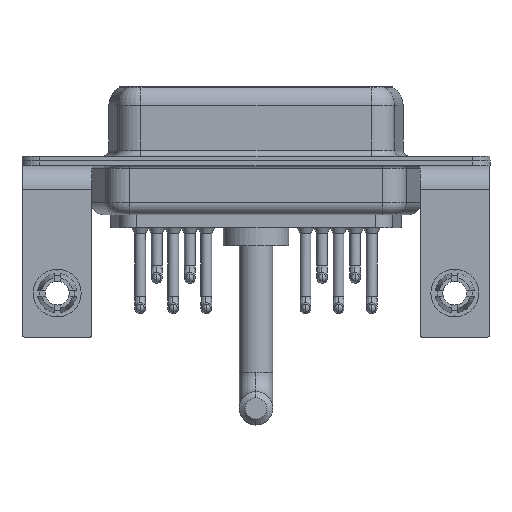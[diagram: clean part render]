
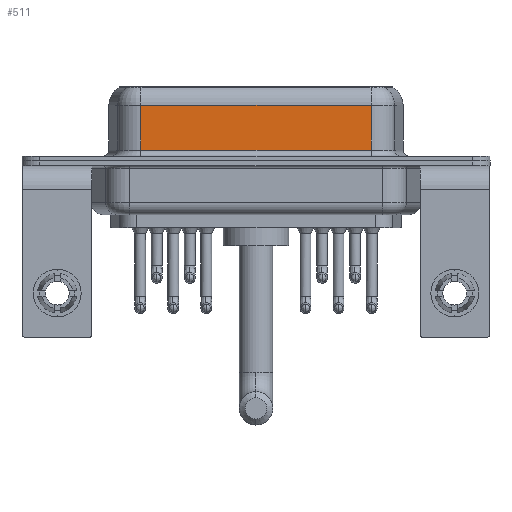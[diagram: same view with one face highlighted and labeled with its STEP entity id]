
A CAD part, front view. The second image highlights one B-rep face of the part: STEP entity #511.
In plain terms, the highlighted planar face has unit normal (0, -1, 0).
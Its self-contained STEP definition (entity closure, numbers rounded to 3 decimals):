
#489 = EDGE_CURVE ( 'NONE', #3411, #7464, #17789, .T. ) ;
#511 = ADVANCED_FACE ( 'NONE', ( #16624 ), #15010, .F. ) ;
#990 = DIRECTION ( 'NONE',  ( 0., 0., -1. ) ) ;
#3123 = CARTESIAN_POINT ( 'NONE',  ( 7.013, -3.95, 4.65 ) ) ;
#3186 = DIRECTION ( 'NONE',  ( -1., 0., 0. ) ) ;
#3411 = VERTEX_POINT ( 'NONE', #3600 ) ;
#3550 = LINE ( 'NONE', #10042, #9897 ) ;
#3600 = CARTESIAN_POINT ( 'NONE',  ( 26.287, -3.95, 4.65 ) ) ;
#4294 = CARTESIAN_POINT ( 'NONE',  ( 7.013, -3.95, 6.4 ) ) ;
#4353 = ORIENTED_EDGE ( 'NONE', *, *, #9801, .F. ) ;
#4501 = CARTESIAN_POINT ( 'NONE',  ( 26.287, -3.95, 0.9 ) ) ;
#4863 = VECTOR ( 'NONE', #18036, 1000. ) ;
#5790 = ORIENTED_EDGE ( 'NONE', *, *, #489, .T. ) ;
#6959 = CARTESIAN_POINT ( 'NONE',  ( 26.287, -3.95, 0.9 ) ) ;
#7464 = VERTEX_POINT ( 'NONE', #3123 ) ;
#9180 = VERTEX_POINT ( 'NONE', #14557 ) ;
#9801 = EDGE_CURVE ( 'NONE', #3411, #19816, #3550, .T. ) ;
#9897 = VECTOR ( 'NONE', #16562, 1000. ) ;
#9956 = VECTOR ( 'NONE', #990, 1000. ) ;
#10042 = CARTESIAN_POINT ( 'NONE',  ( 26.287, -3.95, 6.4 ) ) ;
#12236 = EDGE_LOOP ( 'NONE', ( #4353, #5790, #18954, #19613 ) ) ;
#14557 = CARTESIAN_POINT ( 'NONE',  ( 7.013, -3.95, 0.9 ) ) ;
#15010 = PLANE ( 'NONE',  #19242 ) ;
#15192 = VECTOR ( 'NONE', #3186, 1000. ) ;
#15430 = DIRECTION ( 'NONE',  ( 0., 0., 1. ) ) ;
#15496 = LINE ( 'NONE', #4294, #9956 ) ;
#16562 = DIRECTION ( 'NONE',  ( 0., 0., -1. ) ) ;
#16624 = FACE_OUTER_BOUND ( 'NONE', #12236, .T. ) ;
#16874 = LINE ( 'NONE', #6959, #4863 ) ;
#16921 = EDGE_CURVE ( 'NONE', #7464, #9180, #15496, .T. ) ;
#16940 = CARTESIAN_POINT ( 'NONE',  ( 26.287, -3.95, 6.4 ) ) ;
#17222 = EDGE_CURVE ( 'NONE', #9180, #19816, #16874, .T. ) ;
#17789 = LINE ( 'NONE', #18100, #15192 ) ;
#18036 = DIRECTION ( 'NONE',  ( 1., 0., 0. ) ) ;
#18100 = CARTESIAN_POINT ( 'NONE',  ( 26.287, -3.95, 4.65 ) ) ;
#18954 = ORIENTED_EDGE ( 'NONE', *, *, #16921, .T. ) ;
#19242 = AXIS2_PLACEMENT_3D ( 'NONE', #16940, #20012, #15430 ) ;
#19613 = ORIENTED_EDGE ( 'NONE', *, *, #17222, .T. ) ;
#19816 = VERTEX_POINT ( 'NONE', #4501 ) ;
#20012 = DIRECTION ( 'NONE',  ( 0., 1., 0. ) ) ;
